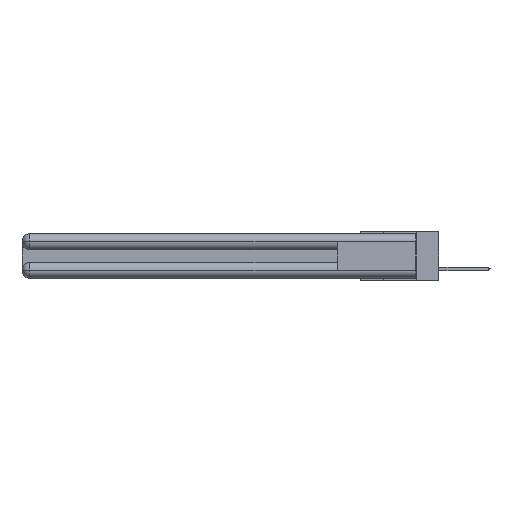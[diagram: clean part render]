
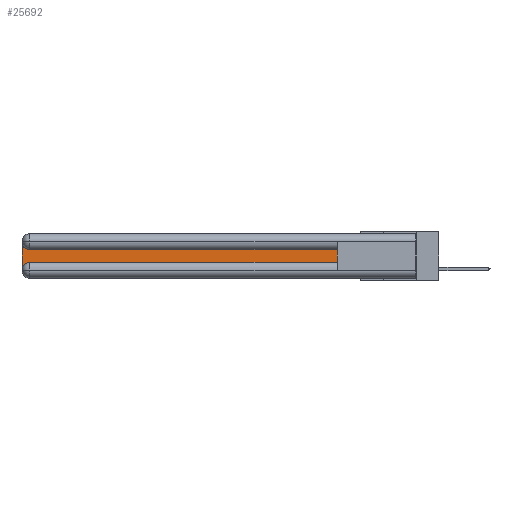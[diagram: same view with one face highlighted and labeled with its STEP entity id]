
A CAD part, left-side view. The second image highlights one B-rep face of the part: STEP entity #25692.
In plain terms, the highlighted planar face has unit normal (-1, 0, 0).
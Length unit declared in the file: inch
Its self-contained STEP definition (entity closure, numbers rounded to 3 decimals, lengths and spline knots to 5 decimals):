
#136 = EDGE_CURVE ( 'NONE', #3994, #19436, #8764, .T. ) ;
#153 = EDGE_CURVE ( 'NONE', #6525, #13461, #28973, .T. ) ;
#381 = ORIENTED_EDGE ( 'NONE', *, *, #15351, .T. ) ;
#690 = PLANE ( 'NONE',  #25837 ) ;
#1444 = VECTOR ( 'NONE', #25741, 39.37008 ) ;
#1576 = ORIENTED_EDGE ( 'NONE', *, *, #14876, .T. ) ;
#2527 = CARTESIAN_POINT ( 'NONE',  ( 0.075, 0.6, -0.2175 ) ) ;
#2771 = DIRECTION ( 'NONE',  ( 1., 0., 0. ) ) ;
#3563 = DIRECTION ( 'NONE',  ( 0., 0., -1. ) ) ;
#3994 = VERTEX_POINT ( 'NONE', #4112 ) ;
#4112 = CARTESIAN_POINT ( 'NONE',  ( 0.075, 3., -0.2775 ) ) ;
#6275 = AXIS2_PLACEMENT_3D ( 'NONE', #29686, #2771, #27366 ) ;
#6444 = CIRCLE ( 'NONE', #6275, 0.06 ) ;
#6525 = VERTEX_POINT ( 'NONE', #28543 ) ;
#7209 = DIRECTION ( 'NONE',  ( 0., -1., 0. ) ) ;
#7467 = CARTESIAN_POINT ( 'NONE',  ( 0.075, 2.94, -0.2775 ) ) ;
#7867 = VECTOR ( 'NONE', #14195, 39.37008 ) ;
#8051 = CARTESIAN_POINT ( 'NONE',  ( 0.075, 3., -0.1225 ) ) ;
#8228 = AXIS2_PLACEMENT_3D ( 'NONE', #7467, #29516, #29305 ) ;
#8700 = CARTESIAN_POINT ( 'NONE',  ( 0.075, 2.94, -0.1225 ) ) ;
#8764 = CIRCLE ( 'NONE', #8228, 0.06 ) ;
#9715 = EDGE_CURVE ( 'NONE', #19436, #19724, #28788, .T. ) ;
#10306 = VECTOR ( 'NONE', #17055, 39.37008 ) ;
#10824 = CARTESIAN_POINT ( 'NONE',  ( 0.075, 3., -0.2175 ) ) ;
#11985 = CARTESIAN_POINT ( 'NONE',  ( 0.075, 3., -0.0625 ) ) ;
#12657 = DIRECTION ( 'NONE',  ( 1., 0., 0. ) ) ;
#13010 = ORIENTED_EDGE ( 'NONE', *, *, #136, .T. ) ;
#13461 = VERTEX_POINT ( 'NONE', #8700 ) ;
#13659 = LINE ( 'NONE', #10824, #1444 ) ;
#14195 = DIRECTION ( 'NONE',  ( 0., 0., 1. ) ) ;
#14434 = ORIENTED_EDGE ( 'NONE', *, *, #28051, .T. ) ;
#14876 = EDGE_CURVE ( 'NONE', #19724, #6525, #28832, .T. ) ;
#15351 = EDGE_CURVE ( 'NONE', #31360, #3994, #13659, .T. ) ;
#17055 = DIRECTION ( 'NONE',  ( 0., 1., 0. ) ) ;
#17323 = ORIENTED_EDGE ( 'NONE', *, *, #9715, .T. ) ;
#18543 = VECTOR ( 'NONE', #7209, 39.37008 ) ;
#19436 = VERTEX_POINT ( 'NONE', #23806 ) ;
#19724 = VERTEX_POINT ( 'NONE', #2527 ) ;
#23806 = CARTESIAN_POINT ( 'NONE',  ( 0.075, 2.94, -0.2175 ) ) ;
#23984 = CARTESIAN_POINT ( 'NONE',  ( 0.075, 0.6, -0.2175 ) ) ;
#25692 = ADVANCED_FACE ( 'NONE', ( #31325 ), #690, .F. ) ;
#25741 = DIRECTION ( 'NONE',  ( 0., 0., -1. ) ) ;
#25837 = AXIS2_PLACEMENT_3D ( 'NONE', #8051, #12657, #3563 ) ;
#26855 = CARTESIAN_POINT ( 'NONE',  ( 0.075, 0.6, -0.1225 ) ) ;
#27366 = DIRECTION ( 'NONE',  ( 0., 0., -1. ) ) ;
#28051 = EDGE_CURVE ( 'NONE', #13461, #31360, #6444, .T. ) ;
#28543 = CARTESIAN_POINT ( 'NONE',  ( 0.075, 0.6, -0.1225 ) ) ;
#28788 = LINE ( 'NONE', #23984, #18543 ) ;
#28832 = LINE ( 'NONE', #31224, #7867 ) ;
#28973 = LINE ( 'NONE', #26855, #10306 ) ;
#29105 = EDGE_LOOP ( 'NONE', ( #29877, #14434, #381, #13010, #17323, #1576 ) ) ;
#29305 = DIRECTION ( 'NONE',  ( 0., 0., -1. ) ) ;
#29516 = DIRECTION ( 'NONE',  ( 1., 0., 0. ) ) ;
#29686 = CARTESIAN_POINT ( 'NONE',  ( 0.075, 2.94, -0.0625 ) ) ;
#29877 = ORIENTED_EDGE ( 'NONE', *, *, #153, .T. ) ;
#31224 = CARTESIAN_POINT ( 'NONE',  ( 0.075, 0.6, -0.2175 ) ) ;
#31325 = FACE_OUTER_BOUND ( 'NONE', #29105, .T. ) ;
#31360 = VERTEX_POINT ( 'NONE', #11985 ) ;
